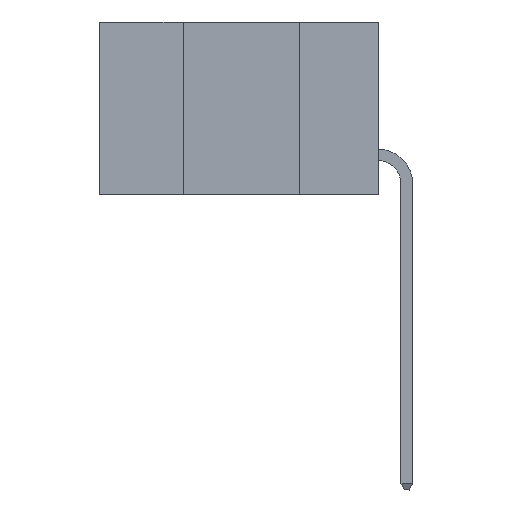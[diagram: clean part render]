
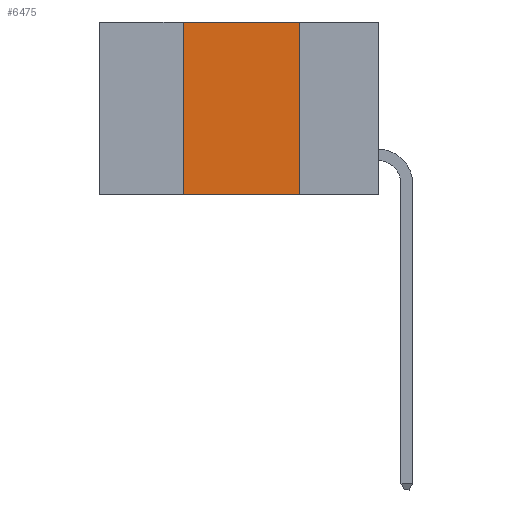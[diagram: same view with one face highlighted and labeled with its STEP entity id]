
A CAD part, left-side view. The second image highlights one B-rep face of the part: STEP entity #6475.
In plain terms, the highlighted planar face has unit normal (-1, 0, 0).
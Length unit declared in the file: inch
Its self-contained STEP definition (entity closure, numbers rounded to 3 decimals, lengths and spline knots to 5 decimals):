
#154 = EDGE_CURVE ( 'NONE', #8989, #4613, #12246, .T. ) ;
#967 = AXIS2_PLACEMENT_3D ( 'NONE', #13082, #2396, #11723 ) ;
#1085 = VECTOR ( 'NONE', #6359, 39.37008 ) ;
#1208 = CARTESIAN_POINT ( 'NONE',  ( 0., 0.6, 0. ) ) ;
#1630 = DIRECTION ( 'NONE',  ( 0., -1., 0. ) ) ;
#2392 = ORIENTED_EDGE ( 'NONE', *, *, #4535, .F. ) ;
#2396 = DIRECTION ( 'NONE',  ( 1., 0., 0. ) ) ;
#2462 = EDGE_CURVE ( 'NONE', #8989, #12469, #11150, .T. ) ;
#2530 = PLANE ( 'NONE',  #967 ) ;
#3275 = DIRECTION ( 'NONE',  ( 0., -1., 0. ) ) ;
#4535 = EDGE_CURVE ( 'NONE', #4613, #7965, #8539, .T. ) ;
#4613 = VERTEX_POINT ( 'NONE', #7830 ) ;
#4758 = CARTESIAN_POINT ( 'NONE',  ( 0., 0.17, -0.37 ) ) ;
#4802 = VECTOR ( 'NONE', #8115, 39.37008 ) ;
#4869 = CARTESIAN_POINT ( 'NONE',  ( 0., 0.42, -0.37 ) ) ;
#5026 = CARTESIAN_POINT ( 'NONE',  ( 0., 0.6, -0.37 ) ) ;
#6019 = ORIENTED_EDGE ( 'NONE', *, *, #7655, .F. ) ;
#6359 = DIRECTION ( 'NONE',  ( 0., 0., -1. ) ) ;
#6475 = ADVANCED_FACE ( 'NONE', ( #11986 ), #2530, .F. ) ;
#6994 = ORIENTED_EDGE ( 'NONE', *, *, #154, .F. ) ;
#7105 = VECTOR ( 'NONE', #3275, 39.37008 ) ;
#7655 = EDGE_CURVE ( 'NONE', #7965, #12469, #13565, .T. ) ;
#7830 = CARTESIAN_POINT ( 'NONE',  ( 0., 0.42, 0. ) ) ;
#7965 = VERTEX_POINT ( 'NONE', #11297 ) ;
#8115 = DIRECTION ( 'NONE',  ( 0., 0., 1. ) ) ;
#8539 = LINE ( 'NONE', #1208, #7105 ) ;
#8989 = VERTEX_POINT ( 'NONE', #10304 ) ;
#10304 = CARTESIAN_POINT ( 'NONE',  ( 0., 0.42, -0.37 ) ) ;
#10706 = CARTESIAN_POINT ( 'NONE',  ( 0., 0.17, -0.37 ) ) ;
#11150 = LINE ( 'NONE', #5026, #12199 ) ;
#11297 = CARTESIAN_POINT ( 'NONE',  ( 0., 0.17, 0. ) ) ;
#11390 = ORIENTED_EDGE ( 'NONE', *, *, #2462, .T. ) ;
#11723 = DIRECTION ( 'NONE',  ( 0., 0., -1. ) ) ;
#11986 = FACE_OUTER_BOUND ( 'NONE', #12766, .T. ) ;
#12199 = VECTOR ( 'NONE', #1630, 39.37008 ) ;
#12246 = LINE ( 'NONE', #4869, #4802 ) ;
#12469 = VERTEX_POINT ( 'NONE', #4758 ) ;
#12766 = EDGE_LOOP ( 'NONE', ( #6019, #2392, #6994, #11390 ) ) ;
#13082 = CARTESIAN_POINT ( 'NONE',  ( 0., 0.6, 0. ) ) ;
#13565 = LINE ( 'NONE', #10706, #1085 ) ;
